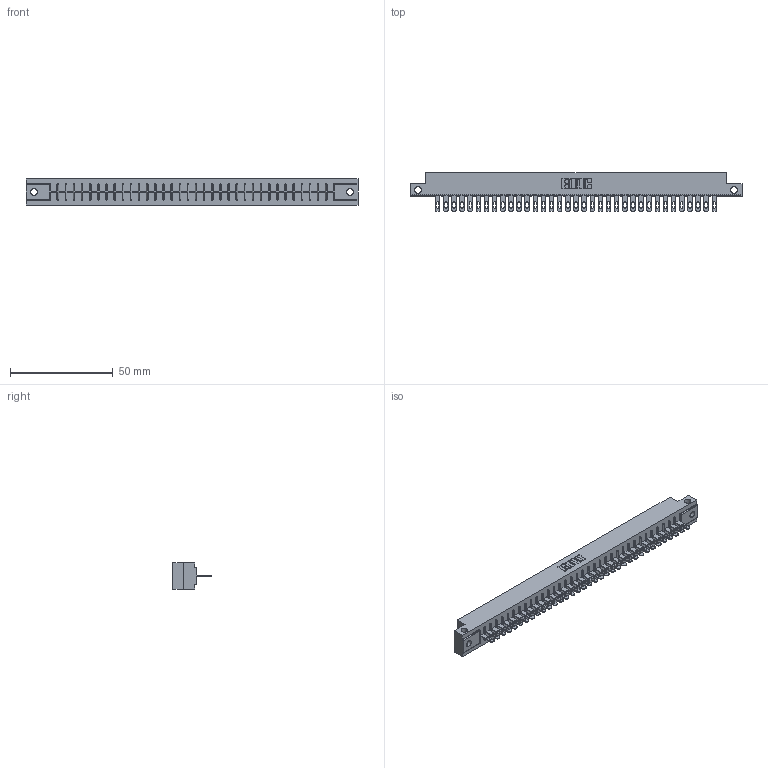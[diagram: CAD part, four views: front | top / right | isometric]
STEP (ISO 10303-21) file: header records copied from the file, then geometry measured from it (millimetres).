
FILE_DESCRIPTION (( 'STEP AP203' ), '1' );
FILE_NAME ('316-035-400-112.STEP', '2020-09-23T04:33:23', ( '' ), ( '' ), 'SwSTEP 2.0', 'SolidWorks 2020', '' );
FILE_SCHEMA (( 'CONFIG_CONTROL_DESIGN' ));
Length unit declared in the file: inch
Products named in the file (3): 316-035-400-112; 306-290-001_100; 306 Part_.128 Dia
Assembly tree (36 placements, depth 2):
  316-035-400-112
    306 Part_.128 Dia
    306-290-001_100  x35
Bounding box: 161.7 x 18.87 x 12.7 mm (x, y, z)
Volume: 17735.2 mm3; surface area: 18767.3 mm2
Topology: 36 solids, 36 shells, 2788 faces, 7877 edges, 5058 vertices
Faces by surface type: plane 1818, cylinder 830, sphere 140
Entity records: 34116 total; most frequent: CARTESIAN_POINT 5776, ORIENTED_EDGE 5682, DIRECTION 5635, EDGE_CURVE 2841, LINE 2201, VECTOR 2201, VERTEX_POINT 1794, AXIS2_PLACEMENT_3D 1717
